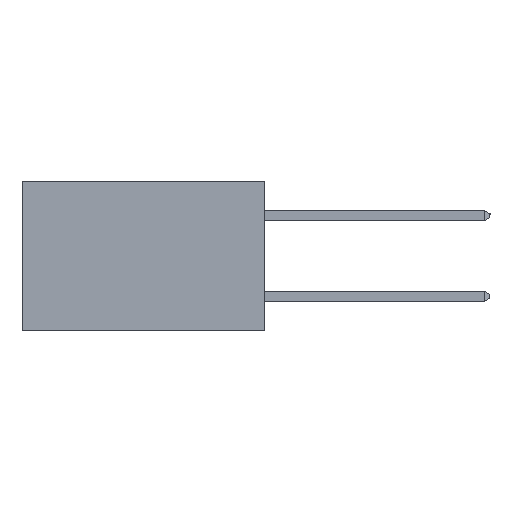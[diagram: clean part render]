
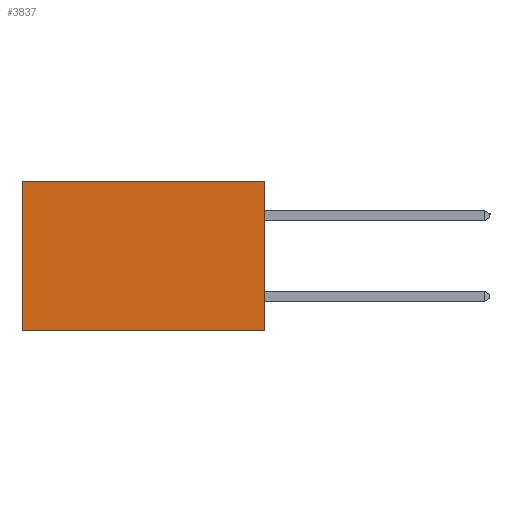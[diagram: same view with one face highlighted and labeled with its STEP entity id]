
A CAD part, left-side view. The second image highlights one B-rep face of the part: STEP entity #3837.
In plain terms, the highlighted planar face has unit normal (-1, 0, 0).
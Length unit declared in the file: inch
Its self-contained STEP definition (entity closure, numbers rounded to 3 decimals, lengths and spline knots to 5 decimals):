
#946 = AXIS2_PLACEMENT_3D ( 'NONE', #8286, #23759, #2392 ) ;
#1767 = LINE ( 'NONE', #10966, #10657 ) ;
#2148 = PLANE ( 'NONE',  #946 ) ;
#2392 = DIRECTION ( 'NONE',  ( 0., 0., -1. ) ) ;
#3091 = EDGE_CURVE ( 'NONE', #6843, #20952, #5583, .T. ) ;
#3234 = CARTESIAN_POINT ( 'NONE',  ( 0.2615, 0.6, -0.37 ) ) ;
#3476 = VECTOR ( 'NONE', #12936, 39.37008 ) ;
#3537 = DIRECTION ( 'NONE',  ( 0., 1., 0. ) ) ;
#3837 = ADVANCED_FACE ( 'NONE', ( #10073 ), #2148, .F. ) ;
#5583 = LINE ( 'NONE', #13348, #22158 ) ;
#5819 = ORIENTED_EDGE ( 'NONE', *, *, #3091, .F. ) ;
#6843 = VERTEX_POINT ( 'NONE', #7118 ) ;
#7118 = CARTESIAN_POINT ( 'NONE',  ( 0.2615, 0., -0.37 ) ) ;
#7175 = VECTOR ( 'NONE', #20703, 39.37008 ) ;
#8286 = CARTESIAN_POINT ( 'NONE',  ( 0.2615, 0., -0.37 ) ) ;
#8817 = EDGE_LOOP ( 'NONE', ( #10619, #5819, #14737, #12221 ) ) ;
#9969 = CARTESIAN_POINT ( 'NONE',  ( 0.2615, 0., 0. ) ) ;
#10073 = FACE_OUTER_BOUND ( 'NONE', #8817, .T. ) ;
#10619 = ORIENTED_EDGE ( 'NONE', *, *, #15453, .T. ) ;
#10657 = VECTOR ( 'NONE', #17379, 39.37008 ) ;
#10966 = CARTESIAN_POINT ( 'NONE',  ( 0.2615, 0., 0. ) ) ;
#12221 = ORIENTED_EDGE ( 'NONE', *, *, #24233, .T. ) ;
#12862 = CARTESIAN_POINT ( 'NONE',  ( 0.2615, 0.6, -0.37 ) ) ;
#12936 = DIRECTION ( 'NONE',  ( 0., 0., -1. ) ) ;
#13154 = LINE ( 'NONE', #14833, #7175 ) ;
#13348 = CARTESIAN_POINT ( 'NONE',  ( 0.2615, 0., -0.37 ) ) ;
#13365 = VERTEX_POINT ( 'NONE', #9969 ) ;
#14178 = CARTESIAN_POINT ( 'NONE',  ( 0.2615, 0.6, 0. ) ) ;
#14737 = ORIENTED_EDGE ( 'NONE', *, *, #15860, .F. ) ;
#14833 = CARTESIAN_POINT ( 'NONE',  ( 0.2615, 0., -0.37 ) ) ;
#15362 = LINE ( 'NONE', #3234, #3476 ) ;
#15453 = EDGE_CURVE ( 'NONE', #19700, #20952, #15362, .T. ) ;
#15860 = EDGE_CURVE ( 'NONE', #13365, #6843, #13154, .T. ) ;
#17379 = DIRECTION ( 'NONE',  ( 0., 1., 0. ) ) ;
#19700 = VERTEX_POINT ( 'NONE', #14178 ) ;
#20703 = DIRECTION ( 'NONE',  ( 0., 0., -1. ) ) ;
#20952 = VERTEX_POINT ( 'NONE', #12862 ) ;
#22158 = VECTOR ( 'NONE', #3537, 39.37008 ) ;
#23759 = DIRECTION ( 'NONE',  ( 1., 0., 0. ) ) ;
#24233 = EDGE_CURVE ( 'NONE', #13365, #19700, #1767, .T. ) ;
